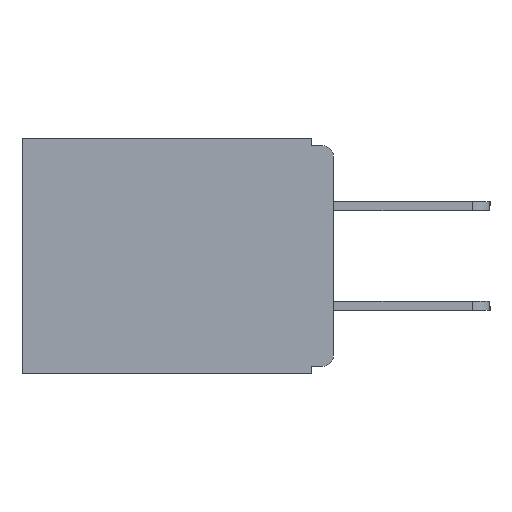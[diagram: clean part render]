
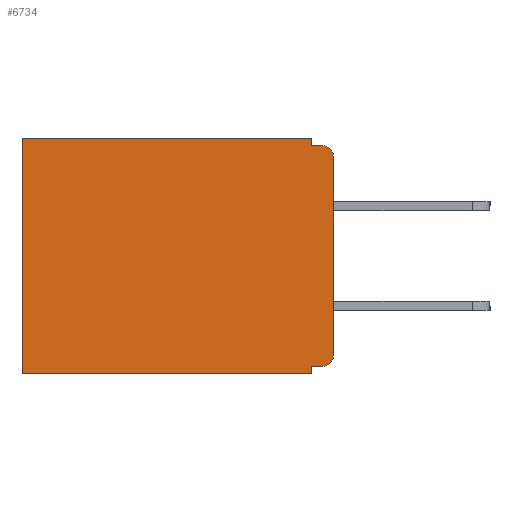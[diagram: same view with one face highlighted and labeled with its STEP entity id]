
A CAD part, left-side view. The second image highlights one B-rep face of the part: STEP entity #6734.
In plain terms, the highlighted planar face has unit normal (-1, 0, 0).
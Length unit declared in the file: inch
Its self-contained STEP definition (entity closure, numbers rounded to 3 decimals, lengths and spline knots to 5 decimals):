
#406 = EDGE_CURVE ( 'NONE', #18413, #29498, #7668, .T. ) ;
#779 = VECTOR ( 'NONE', #17731, 39.37008 ) ;
#833 = VECTOR ( 'NONE', #27538, 39.37008 ) ;
#905 = VECTOR ( 'NONE', #12456, 39.37008 ) ;
#1568 = DIRECTION ( 'NONE',  ( 0., 0., -1. ) ) ;
#1739 = CARTESIAN_POINT ( 'NONE',  ( 0.3, 0.015, -0.025 ) ) ;
#1775 = DIRECTION ( 'NONE',  ( -1., 0., 0. ) ) ;
#1814 = AXIS2_PLACEMENT_3D ( 'NONE', #28325, #28059, #28053 ) ;
#1839 = EDGE_CURVE ( 'NONE', #9740, #29985, #18091, .T. ) ;
#1970 = VECTOR ( 'NONE', #2914, 39.37008 ) ;
#2541 = VERTEX_POINT ( 'NONE', #12254 ) ;
#2914 = DIRECTION ( 'NONE',  ( 0., 0., -1. ) ) ;
#3998 = VERTEX_POINT ( 'NONE', #20812 ) ;
#4518 = CARTESIAN_POINT ( 'NONE',  ( 0.3, 0.015, -0.32 ) ) ;
#4766 = LINE ( 'NONE', #25934, #16863 ) ;
#4828 = EDGE_CURVE ( 'NONE', #28401, #25638, #18505, .T. ) ;
#6443 = CARTESIAN_POINT ( 'NONE',  ( 0.3, 0., -0.33 ) ) ;
#6734 = ADVANCED_FACE ( 'NONE', ( #15825 ), #28455, .F. ) ;
#7496 = CARTESIAN_POINT ( 'NONE',  ( 0.3, 0., -0.33 ) ) ;
#7668 = LINE ( 'NONE', #13535, #1970 ) ;
#8047 = EDGE_CURVE ( 'NONE', #29498, #2541, #17238, .T. ) ;
#9252 = EDGE_CURVE ( 'NONE', #3998, #25638, #16890, .T. ) ;
#9385 = AXIS2_PLACEMENT_3D ( 'NONE', #1739, #1775, #1568 ) ;
#9582 = EDGE_CURVE ( 'NONE', #28401, #29985, #24747, .T. ) ;
#9645 = EDGE_CURVE ( 'NONE', #19329, #2541, #4766, .T. ) ;
#9695 = ORIENTED_EDGE ( 'NONE', *, *, #4828, .T. ) ;
#9740 = VERTEX_POINT ( 'NONE', #4518 ) ;
#9767 = VECTOR ( 'NONE', #12506, 39.37008 ) ;
#10124 = VECTOR ( 'NONE', #21881, 39.37008 ) ;
#11226 = CARTESIAN_POINT ( 'NONE',  ( 0.3, 0.031, 0. ) ) ;
#11437 = CARTESIAN_POINT ( 'NONE',  ( 0.3, 0., -0.305 ) ) ;
#11827 = ORIENTED_EDGE ( 'NONE', *, *, #24584, .F. ) ;
#12254 = CARTESIAN_POINT ( 'NONE',  ( 0.3, 0.437, -0.33 ) ) ;
#12456 = DIRECTION ( 'NONE',  ( 0., 1., 0. ) ) ;
#12506 = DIRECTION ( 'NONE',  ( 0., -1., 0. ) ) ;
#12712 = ORIENTED_EDGE ( 'NONE', *, *, #8047, .F. ) ;
#13535 = CARTESIAN_POINT ( 'NONE',  ( 0.3, 0.031, -0.33 ) ) ;
#13728 = LINE ( 'NONE', #25127, #833 ) ;
#13979 = ORIENTED_EDGE ( 'NONE', *, *, #406, .F. ) ;
#14407 = LINE ( 'NONE', #15347, #779 ) ;
#15347 = CARTESIAN_POINT ( 'NONE',  ( 0.3, 0.031, 0. ) ) ;
#15825 = FACE_OUTER_BOUND ( 'NONE', #28117, .T. ) ;
#16255 = DIRECTION ( 'NONE',  ( 0., 0., -1. ) ) ;
#16863 = VECTOR ( 'NONE', #16255, 39.37008 ) ;
#16890 = LINE ( 'NONE', #29309, #9767 ) ;
#17238 = LINE ( 'NONE', #7496, #10124 ) ;
#17731 = DIRECTION ( 'NONE',  ( 0., 0., -1. ) ) ;
#18091 = CIRCLE ( 'NONE', #1814, 0.015 ) ;
#18346 = VECTOR ( 'NONE', #20865, 39.37008 ) ;
#18413 = VERTEX_POINT ( 'NONE', #29219 ) ;
#18505 = CIRCLE ( 'NONE', #9385, 0.015 ) ;
#19041 = ORIENTED_EDGE ( 'NONE', *, *, #9582, .F. ) ;
#19329 = VERTEX_POINT ( 'NONE', #23245 ) ;
#19543 = CARTESIAN_POINT ( 'NONE',  ( 0.3, 0.015, -0.01 ) ) ;
#20132 = LINE ( 'NONE', #24308, #905 ) ;
#20812 = CARTESIAN_POINT ( 'NONE',  ( 0.3, 0.031, -0.01 ) ) ;
#20865 = DIRECTION ( 'NONE',  ( 0., 0., -1. ) ) ;
#21219 = ORIENTED_EDGE ( 'NONE', *, *, #9252, .F. ) ;
#21278 = DIRECTION ( 'NONE',  ( 1., 0., 0. ) ) ;
#21881 = DIRECTION ( 'NONE',  ( 0., 1., 0. ) ) ;
#22624 = ORIENTED_EDGE ( 'NONE', *, *, #31158, .F. ) ;
#23245 = CARTESIAN_POINT ( 'NONE',  ( 0.3, 0.437, 0. ) ) ;
#24308 = CARTESIAN_POINT ( 'NONE',  ( 0.3, 0., 0. ) ) ;
#24381 = ORIENTED_EDGE ( 'NONE', *, *, #9645, .T. ) ;
#24584 = EDGE_CURVE ( 'NONE', #29951, #3998, #14407, .T. ) ;
#24721 = CARTESIAN_POINT ( 'NONE',  ( 0.3, 0., -0.025 ) ) ;
#24747 = LINE ( 'NONE', #6443, #18346 ) ;
#25127 = CARTESIAN_POINT ( 'NONE',  ( 0.3, 0., -0.32 ) ) ;
#25505 = ORIENTED_EDGE ( 'NONE', *, *, #30274, .T. ) ;
#25638 = VERTEX_POINT ( 'NONE', #19543 ) ;
#25934 = CARTESIAN_POINT ( 'NONE',  ( 0.3, 0.437, -0.33 ) ) ;
#26126 = CARTESIAN_POINT ( 'NONE',  ( 0.3, 0., -0.33 ) ) ;
#26457 = CARTESIAN_POINT ( 'NONE',  ( 0.3, 0.031, -0.33 ) ) ;
#26551 = ORIENTED_EDGE ( 'NONE', *, *, #1839, .T. ) ;
#27538 = DIRECTION ( 'NONE',  ( 0., 1., 0. ) ) ;
#28053 = DIRECTION ( 'NONE',  ( 0., 0., -1. ) ) ;
#28059 = DIRECTION ( 'NONE',  ( -1., 0., 0. ) ) ;
#28117 = EDGE_LOOP ( 'NONE', ( #19041, #9695, #21219, #11827, #25505, #24381, #12712, #13979, #22624, #26551 ) ) ;
#28325 = CARTESIAN_POINT ( 'NONE',  ( 0.3, 0.015, -0.305 ) ) ;
#28401 = VERTEX_POINT ( 'NONE', #24721 ) ;
#28455 = PLANE ( 'NONE',  #30391 ) ;
#29219 = CARTESIAN_POINT ( 'NONE',  ( 0.3, 0.031, -0.32 ) ) ;
#29309 = CARTESIAN_POINT ( 'NONE',  ( 0.3, 0., -0.01 ) ) ;
#29498 = VERTEX_POINT ( 'NONE', #26457 ) ;
#29951 = VERTEX_POINT ( 'NONE', #11226 ) ;
#29985 = VERTEX_POINT ( 'NONE', #11437 ) ;
#30274 = EDGE_CURVE ( 'NONE', #29951, #19329, #20132, .T. ) ;
#30391 = AXIS2_PLACEMENT_3D ( 'NONE', #26126, #21278, #31159 ) ;
#31158 = EDGE_CURVE ( 'NONE', #9740, #18413, #13728, .T. ) ;
#31159 = DIRECTION ( 'NONE',  ( 0., 0., -1. ) ) ;
